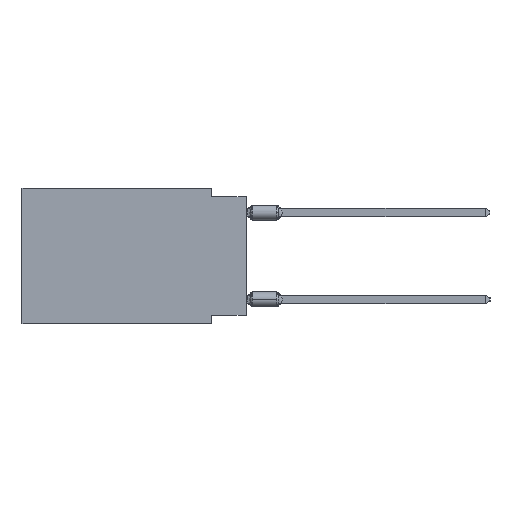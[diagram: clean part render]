
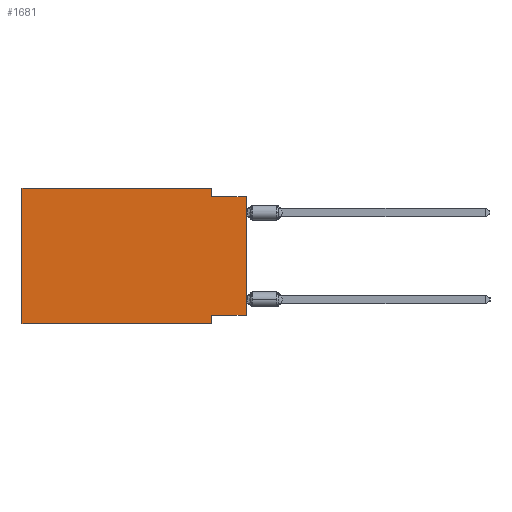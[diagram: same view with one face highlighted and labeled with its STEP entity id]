
A CAD part, left-side view. The second image highlights one B-rep face of the part: STEP entity #1681.
In plain terms, the highlighted planar face has unit normal (-1, 0, 0).
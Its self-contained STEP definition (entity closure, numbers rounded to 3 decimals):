
#36 = DIRECTION ( 'NONE',  ( 1., 0., 0. ) ) ;
#490 = CARTESIAN_POINT ( 'NONE',  ( 0., 16.383, 0. ) ) ;
#1681 = ADVANCED_FACE ( 'NONE', ( #35011 ), #42544, .F. ) ;
#1867 = CARTESIAN_POINT ( 'NONE',  ( 0., 0., -0.635 ) ) ;
#2136 = VERTEX_POINT ( 'NONE', #1867 ) ;
#3207 = DIRECTION ( 'NONE',  ( 0., 0., -1. ) ) ;
#5919 = DIRECTION ( 'NONE',  ( 0., 1., 0. ) ) ;
#6064 = DIRECTION ( 'NONE',  ( 0., -1., 0. ) ) ;
#6484 = VECTOR ( 'NONE', #3207, 1000. ) ;
#7089 = LINE ( 'NONE', #34515, #6484 ) ;
#7366 = DIRECTION ( 'NONE',  ( 0., 0., -1. ) ) ;
#7568 = DIRECTION ( 'NONE',  ( 0., 0., -1. ) ) ;
#8535 = ORIENTED_EDGE ( 'NONE', *, *, #34960, .F. ) ;
#10248 = CARTESIAN_POINT ( 'NONE',  ( 0., 0., 0. ) ) ;
#10278 = EDGE_CURVE ( 'NONE', #16904, #28329, #15530, .T. ) ;
#10286 = CARTESIAN_POINT ( 'NONE',  ( 0., 16.383, 0. ) ) ;
#11227 = ORIENTED_EDGE ( 'NONE', *, *, #27822, .F. ) ;
#11975 = VECTOR ( 'NONE', #18690, 1000. ) ;
#12300 = VECTOR ( 'NONE', #7366, 1000. ) ;
#13025 = VERTEX_POINT ( 'NONE', #42315 ) ;
#13138 = CARTESIAN_POINT ( 'NONE',  ( 0., 0., -0.635 ) ) ;
#15366 = LINE ( 'NONE', #36389, #43777 ) ;
#15530 = LINE ( 'NONE', #30603, #25274 ) ;
#16660 = LINE ( 'NONE', #10248, #22668 ) ;
#16904 = VERTEX_POINT ( 'NONE', #42978 ) ;
#17549 = EDGE_CURVE ( 'NONE', #13025, #32305, #30305, .T. ) ;
#17912 = VECTOR ( 'NONE', #6064, 1000. ) ;
#18317 = CARTESIAN_POINT ( 'NONE',  ( 0., 2.54, -0.635 ) ) ;
#18690 = DIRECTION ( 'NONE',  ( 0., 0., 1. ) ) ;
#21331 = ORIENTED_EDGE ( 'NONE', *, *, #40097, .F. ) ;
#21523 = CARTESIAN_POINT ( 'NONE',  ( 0., 2.54, 0. ) ) ;
#22425 = DIRECTION ( 'NONE',  ( 0., -1., 0. ) ) ;
#22668 = VECTOR ( 'NONE', #31043, 1000. ) ;
#22906 = CARTESIAN_POINT ( 'NONE',  ( 0., 2.54, -9.271 ) ) ;
#24269 = VERTEX_POINT ( 'NONE', #35879 ) ;
#24490 = EDGE_CURVE ( 'NONE', #16904, #2136, #16660, .T. ) ;
#24782 = ORIENTED_EDGE ( 'NONE', *, *, #28651, .T. ) ;
#25274 = VECTOR ( 'NONE', #5919, 1000. ) ;
#25641 = EDGE_CURVE ( 'NONE', #27445, #2136, #37149, .T. ) ;
#27081 = DIRECTION ( 'NONE',  ( 0., -1., 0. ) ) ;
#27445 = VERTEX_POINT ( 'NONE', #18317 ) ;
#27648 = AXIS2_PLACEMENT_3D ( 'NONE', #490, #36, #7568 ) ;
#27822 = EDGE_CURVE ( 'NONE', #32305, #27445, #7089, .T. ) ;
#28175 = LINE ( 'NONE', #42117, #12300 ) ;
#28329 = VERTEX_POINT ( 'NONE', #22906 ) ;
#28651 = EDGE_CURVE ( 'NONE', #24269, #36282, #15366, .T. ) ;
#30305 = LINE ( 'NONE', #34400, #17912 ) ;
#30603 = CARTESIAN_POINT ( 'NONE',  ( 0., 0., -9.271 ) ) ;
#31043 = DIRECTION ( 'NONE',  ( 0., 0., 1. ) ) ;
#31083 = LINE ( 'NONE', #10286, #11975 ) ;
#32305 = VERTEX_POINT ( 'NONE', #21523 ) ;
#33251 = EDGE_LOOP ( 'NONE', ( #38259, #43839, #11227, #42659, #21331, #24782, #8535, #44520 ) ) ;
#34400 = CARTESIAN_POINT ( 'NONE',  ( 0., 16.383, 0. ) ) ;
#34515 = CARTESIAN_POINT ( 'NONE',  ( 0., 2.54, 0. ) ) ;
#34960 = EDGE_CURVE ( 'NONE', #28329, #36282, #28175, .T. ) ;
#35011 = FACE_OUTER_BOUND ( 'NONE', #33251, .T. ) ;
#35879 = CARTESIAN_POINT ( 'NONE',  ( 0., 16.383, -9.906 ) ) ;
#36213 = CARTESIAN_POINT ( 'NONE',  ( 0., 2.54, -9.906 ) ) ;
#36282 = VERTEX_POINT ( 'NONE', #36213 ) ;
#36389 = CARTESIAN_POINT ( 'NONE',  ( 0., 16.383, -9.906 ) ) ;
#37149 = LINE ( 'NONE', #13138, #39210 ) ;
#38259 = ORIENTED_EDGE ( 'NONE', *, *, #24490, .T. ) ;
#39210 = VECTOR ( 'NONE', #27081, 1000. ) ;
#40097 = EDGE_CURVE ( 'NONE', #24269, #13025, #31083, .T. ) ;
#42117 = CARTESIAN_POINT ( 'NONE',  ( 0., 2.54, -9.906 ) ) ;
#42315 = CARTESIAN_POINT ( 'NONE',  ( 0., 16.383, 0. ) ) ;
#42544 = PLANE ( 'NONE',  #27648 ) ;
#42659 = ORIENTED_EDGE ( 'NONE', *, *, #17549, .F. ) ;
#42978 = CARTESIAN_POINT ( 'NONE',  ( 0., 0., -9.271 ) ) ;
#43777 = VECTOR ( 'NONE', #22425, 1000. ) ;
#43839 = ORIENTED_EDGE ( 'NONE', *, *, #25641, .F. ) ;
#44520 = ORIENTED_EDGE ( 'NONE', *, *, #10278, .F. ) ;
